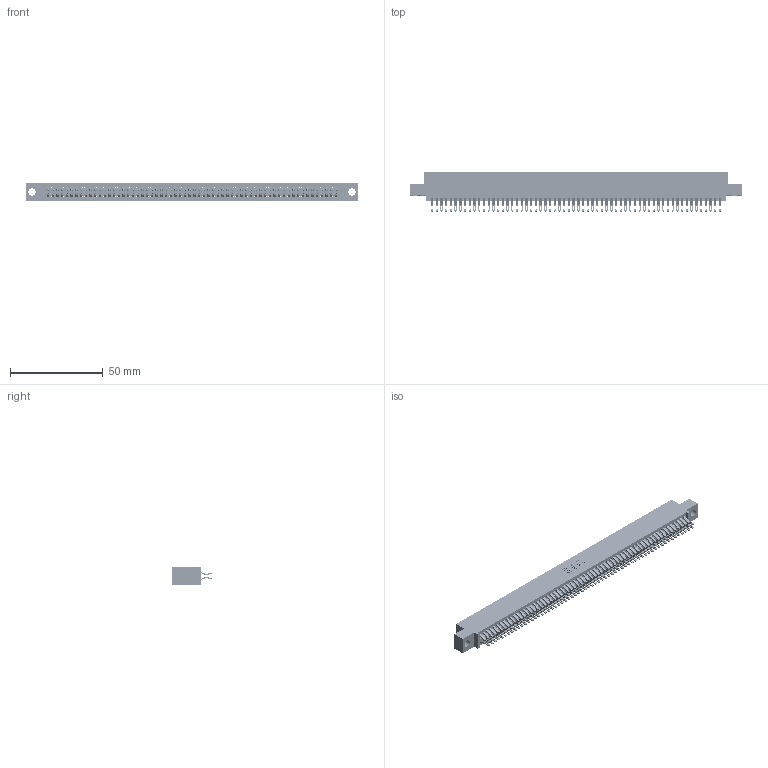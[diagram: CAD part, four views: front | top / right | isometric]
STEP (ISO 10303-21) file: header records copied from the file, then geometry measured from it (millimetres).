
FILE_DESCRIPTION (( 'STEP AP203' ), '1' );
FILE_NAME ('395-124-555-504.STEP', '2021-06-17T22:19:57', ( '' ), ( '' ), 'SwSTEP 2.0', 'SolidWorks 2020', '' );
FILE_SCHEMA (( 'CONFIG_CONTROL_DESIGN' ));
Length unit declared in the file: inch
Products named in the file (3): 345-292-001_555 Tail; 345 Part_0.110 Offset - 0.156 Dia-TI; 395-124-555-504
Assembly tree (125 placements, depth 2):
  395-124-555-504
    345 Part_0.110 Offset - 0.156 Dia-TI
    345-292-001_555 Tail  x124
Bounding box: 178.69 x 21.13 x 9.4 mm (x, y, z)
Volume: 17724 mm3; surface area: 27781.8 mm2
Topology: 125 solids, 125 shells, 7088 faces, 22337 edges, 14890 vertices
Faces by surface type: plane 3942, cylinder 3146
Entity records: 46831 total; most frequent: CARTESIAN_POINT 7872, ORIENTED_EDGE 7774, DIRECTION 6883, EDGE_CURVE 3887, LINE 3487, VECTOR 3487, VERTEX_POINT 2590, AXIS2_PLACEMENT_3D 1698
